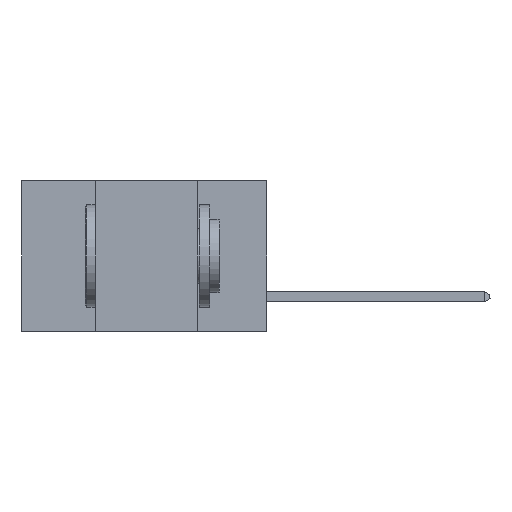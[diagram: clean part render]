
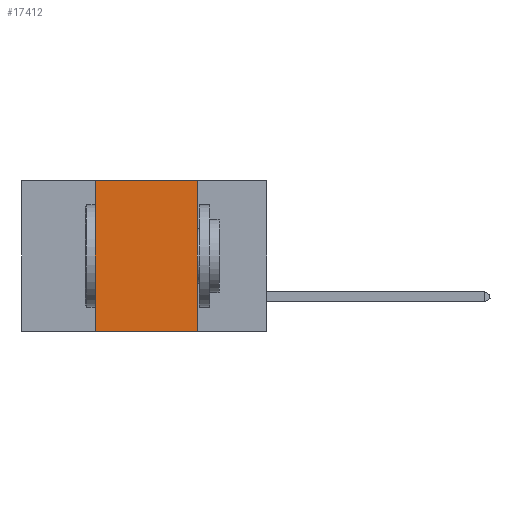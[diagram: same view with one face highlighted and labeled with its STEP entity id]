
A CAD part, left-side view. The second image highlights one B-rep face of the part: STEP entity #17412.
In plain terms, the highlighted planar face has unit normal (-1, 0, 0).
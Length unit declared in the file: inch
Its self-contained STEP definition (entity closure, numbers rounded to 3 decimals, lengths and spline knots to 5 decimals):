
#1538 = PLANE ( 'NONE',  #22518 ) ;
#1708 = DIRECTION ( 'NONE',  ( 0., 0., -1. ) ) ;
#1932 = VERTEX_POINT ( 'NONE', #18518 ) ;
#4579 = VECTOR ( 'NONE', #4660, 39.37008 ) ;
#4660 = DIRECTION ( 'NONE',  ( 0., -1., 0. ) ) ;
#4935 = CARTESIAN_POINT ( 'NONE',  ( 0., 0.42, 0. ) ) ;
#6198 = ORIENTED_EDGE ( 'NONE', *, *, #13456, .F. ) ;
#6942 = EDGE_CURVE ( 'NONE', #1932, #9455, #25920, .T. ) ;
#7817 = CARTESIAN_POINT ( 'NONE',  ( 0., 0.17, 0. ) ) ;
#8001 = CARTESIAN_POINT ( 'NONE',  ( 0., 0.6, 0. ) ) ;
#9433 = VECTOR ( 'NONE', #26743, 39.37008 ) ;
#9455 = VERTEX_POINT ( 'NONE', #15138 ) ;
#9582 = FACE_OUTER_BOUND ( 'NONE', #24772, .T. ) ;
#13004 = DIRECTION ( 'NONE',  ( 0., 0., -1. ) ) ;
#13091 = ORIENTED_EDGE ( 'NONE', *, *, #19028, .F. ) ;
#13313 = VECTOR ( 'NONE', #25979, 39.37008 ) ;
#13456 = EDGE_CURVE ( 'NONE', #20925, #23966, #17707, .T. ) ;
#15138 = CARTESIAN_POINT ( 'NONE',  ( 0., 0.42, 0. ) ) ;
#15621 = CARTESIAN_POINT ( 'NONE',  ( 0., 0.6, -0.37 ) ) ;
#15916 = LINE ( 'NONE', #15621, #4579 ) ;
#16950 = CARTESIAN_POINT ( 'NONE',  ( 0., 0.17, -0.37 ) ) ;
#17412 = ADVANCED_FACE ( 'NONE', ( #9582 ), #1538, .F. ) ;
#17707 = LINE ( 'NONE', #25397, #21599 ) ;
#17828 = LINE ( 'NONE', #19970, #13313 ) ;
#18518 = CARTESIAN_POINT ( 'NONE',  ( 0., 0.42, -0.37 ) ) ;
#19028 = EDGE_CURVE ( 'NONE', #9455, #20925, #17828, .T. ) ;
#19083 = ORIENTED_EDGE ( 'NONE', *, *, #23579, .T. ) ;
#19970 = CARTESIAN_POINT ( 'NONE',  ( 0., 0.6, 0. ) ) ;
#20925 = VERTEX_POINT ( 'NONE', #7817 ) ;
#21599 = VECTOR ( 'NONE', #13004, 39.37008 ) ;
#22518 = AXIS2_PLACEMENT_3D ( 'NONE', #8001, #24315, #1708 ) ;
#23579 = EDGE_CURVE ( 'NONE', #1932, #23966, #15916, .T. ) ;
#23966 = VERTEX_POINT ( 'NONE', #16950 ) ;
#24315 = DIRECTION ( 'NONE',  ( 1., 0., 0. ) ) ;
#24772 = EDGE_LOOP ( 'NONE', ( #6198, #13091, #24954, #19083 ) ) ;
#24954 = ORIENTED_EDGE ( 'NONE', *, *, #6942, .F. ) ;
#25397 = CARTESIAN_POINT ( 'NONE',  ( 0., 0.17, 0. ) ) ;
#25920 = LINE ( 'NONE', #4935, #9433 ) ;
#25979 = DIRECTION ( 'NONE',  ( 0., -1., 0. ) ) ;
#26743 = DIRECTION ( 'NONE',  ( 0., 0., 1. ) ) ;
